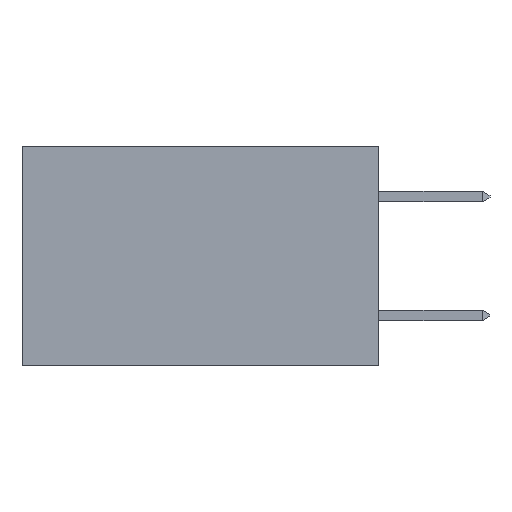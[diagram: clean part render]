
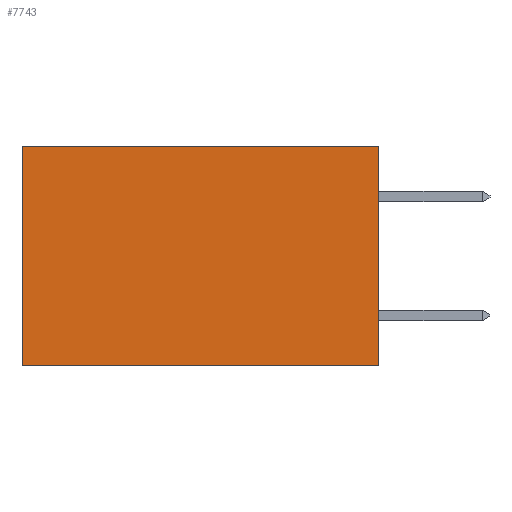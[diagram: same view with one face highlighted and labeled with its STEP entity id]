
A CAD part, left-side view. The second image highlights one B-rep face of the part: STEP entity #7743.
In plain terms, the highlighted planar face has unit normal (-1, 0, 0).
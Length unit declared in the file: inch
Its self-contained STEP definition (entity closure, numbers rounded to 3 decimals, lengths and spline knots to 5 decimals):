
#264 = VERTEX_POINT ( 'NONE', #7347 ) ;
#748 = DIRECTION ( 'NONE',  ( 0., 1., 0. ) ) ;
#899 = PLANE ( 'NONE',  #8069 ) ;
#932 = CARTESIAN_POINT ( 'NONE',  ( 0.298, 0., 0. ) ) ;
#1058 = ORIENTED_EDGE ( 'NONE', *, *, #3446, .T. ) ;
#1096 = EDGE_LOOP ( 'NONE', ( #1058, #1332, #6742, #4275 ) ) ;
#1332 = ORIENTED_EDGE ( 'NONE', *, *, #3513, .F. ) ;
#1410 = VERTEX_POINT ( 'NONE', #2284 ) ;
#1550 = VECTOR ( 'NONE', #748, 39.37008 ) ;
#1626 = CARTESIAN_POINT ( 'NONE',  ( 0.298, 0., 0. ) ) ;
#1753 = DIRECTION ( 'NONE',  ( 0., 0., -1. ) ) ;
#1796 = LINE ( 'NONE', #1626, #1550 ) ;
#2284 = CARTESIAN_POINT ( 'NONE',  ( 0.298, 0., 0. ) ) ;
#2813 = FACE_OUTER_BOUND ( 'NONE', #1096, .T. ) ;
#3129 = CARTESIAN_POINT ( 'NONE',  ( 0.298, 0., -0.37 ) ) ;
#3175 = VECTOR ( 'NONE', #6300, 39.37008 ) ;
#3269 = VERTEX_POINT ( 'NONE', #6725 ) ;
#3446 = EDGE_CURVE ( 'NONE', #7558, #264, #5902, .T. ) ;
#3513 = EDGE_CURVE ( 'NONE', #3269, #264, #5243, .T. ) ;
#3660 = EDGE_CURVE ( 'NONE', #1410, #3269, #5786, .T. ) ;
#4198 = VECTOR ( 'NONE', #5865, 39.37008 ) ;
#4211 = CARTESIAN_POINT ( 'NONE',  ( 0.298, 0.6, 0. ) ) ;
#4275 = ORIENTED_EDGE ( 'NONE', *, *, #4662, .T. ) ;
#4300 = CARTESIAN_POINT ( 'NONE',  ( 0.298, 0.6, 0. ) ) ;
#4662 = EDGE_CURVE ( 'NONE', #1410, #7558, #1796, .T. ) ;
#5243 = LINE ( 'NONE', #3129, #3175 ) ;
#5786 = LINE ( 'NONE', #7742, #9323 ) ;
#5865 = DIRECTION ( 'NONE',  ( 0., 0., -1. ) ) ;
#5902 = LINE ( 'NONE', #4300, #4198 ) ;
#6300 = DIRECTION ( 'NONE',  ( 0., 1., 0. ) ) ;
#6372 = DIRECTION ( 'NONE',  ( 1., 0., 0. ) ) ;
#6725 = CARTESIAN_POINT ( 'NONE',  ( 0.298, 0., -0.37 ) ) ;
#6742 = ORIENTED_EDGE ( 'NONE', *, *, #3660, .F. ) ;
#7347 = CARTESIAN_POINT ( 'NONE',  ( 0.298, 0.6, -0.37 ) ) ;
#7558 = VERTEX_POINT ( 'NONE', #4211 ) ;
#7742 = CARTESIAN_POINT ( 'NONE',  ( 0.298, 0., 0. ) ) ;
#7743 = ADVANCED_FACE ( 'NONE', ( #2813 ), #899, .F. ) ;
#7826 = DIRECTION ( 'NONE',  ( 0., 0., -1. ) ) ;
#8069 = AXIS2_PLACEMENT_3D ( 'NONE', #932, #6372, #1753 ) ;
#9323 = VECTOR ( 'NONE', #7826, 39.37008 ) ;
